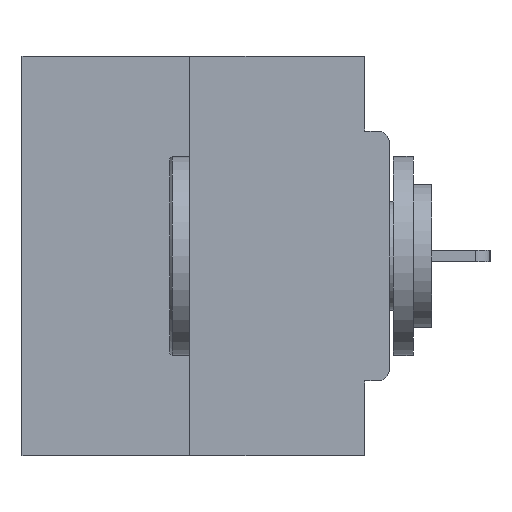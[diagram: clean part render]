
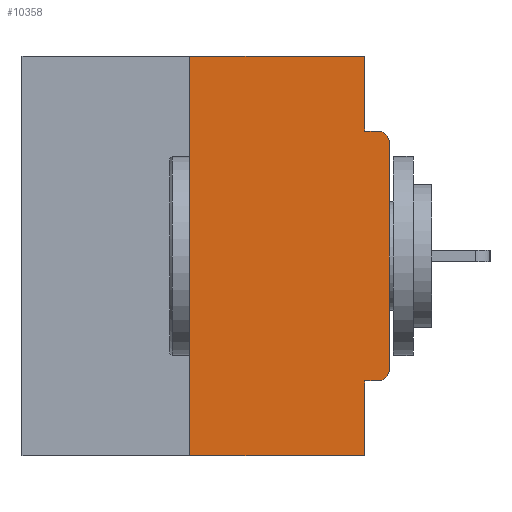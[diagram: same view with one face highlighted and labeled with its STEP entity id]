
A CAD part, left-side view. The second image highlights one B-rep face of the part: STEP entity #10358.
In plain terms, the highlighted planar face has unit normal (-1, 0, 0).
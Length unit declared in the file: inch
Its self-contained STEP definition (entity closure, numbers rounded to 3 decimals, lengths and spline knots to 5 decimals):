
#1266 = DIRECTION ( 'NONE',  ( -1., 0., 0. ) ) ;
#2872 = CARTESIAN_POINT ( 'NONE',  ( 0., 0.46, -0.5 ) ) ;
#3103 = VERTEX_POINT ( 'NONE', #32053 ) ;
#3168 = CARTESIAN_POINT ( 'NONE',  ( 0., 0., -0.4065 ) ) ;
#3614 = ORIENTED_EDGE ( 'NONE', *, *, #15374, .F. ) ;
#3840 = CARTESIAN_POINT ( 'NONE',  ( 0., 0.46, 0. ) ) ;
#3974 = LINE ( 'NONE', #3168, #19905 ) ;
#4709 = AXIS2_PLACEMENT_3D ( 'NONE', #33592, #14643, #36717 ) ;
#5144 = ORIENTED_EDGE ( 'NONE', *, *, #16785, .T. ) ;
#6228 = EDGE_CURVE ( 'NONE', #33086, #18322, #9786, .T. ) ;
#6439 = DIRECTION ( 'NONE',  ( 0., 1., 0. ) ) ;
#6681 = ORIENTED_EDGE ( 'NONE', *, *, #34825, .F. ) ;
#7088 = CARTESIAN_POINT ( 'NONE',  ( 0., 0.031, -0.4065 ) ) ;
#7134 = EDGE_CURVE ( 'NONE', #12726, #3103, #34498, .T. ) ;
#7839 = DIRECTION ( 'NONE',  ( 0., 0., -1. ) ) ;
#7960 = DIRECTION ( 'NONE',  ( 1., 0., 0. ) ) ;
#8054 = VECTOR ( 'NONE', #36622, 39.37008 ) ;
#8109 = PLANE ( 'NONE',  #19011 ) ;
#8117 = CARTESIAN_POINT ( 'NONE',  ( 0., 0.25, -0.5 ) ) ;
#8570 = VECTOR ( 'NONE', #26077, 39.37008 ) ;
#8656 = VERTEX_POINT ( 'NONE', #17662 ) ;
#8841 = CARTESIAN_POINT ( 'NONE',  ( 0., 0.46, 0. ) ) ;
#9786 = LINE ( 'NONE', #16231, #26636 ) ;
#10123 = CARTESIAN_POINT ( 'NONE',  ( 0., 0.031, 0. ) ) ;
#10236 = LINE ( 'NONE', #14665, #34460 ) ;
#10358 = ADVANCED_FACE ( 'NONE', ( #35664 ), #8109, .F. ) ;
#10622 = VERTEX_POINT ( 'NONE', #30970 ) ;
#11756 = VERTEX_POINT ( 'NONE', #8117 ) ;
#12726 = VERTEX_POINT ( 'NONE', #28962 ) ;
#13020 = EDGE_CURVE ( 'NONE', #3103, #8656, #40274, .T. ) ;
#14555 = CARTESIAN_POINT ( 'NONE',  ( 0., 0., -0.0935 ) ) ;
#14591 = ORIENTED_EDGE ( 'NONE', *, *, #39870, .F. ) ;
#14643 = DIRECTION ( 'NONE',  ( -1., 0., 0. ) ) ;
#14665 = CARTESIAN_POINT ( 'NONE',  ( 0., 0.25, 0. ) ) ;
#14798 = CARTESIAN_POINT ( 'NONE',  ( 0., 0.031, 0. ) ) ;
#15153 = EDGE_CURVE ( 'NONE', #22543, #38766, #24403, .T. ) ;
#15210 = CIRCLE ( 'NONE', #15786, 0.015 ) ;
#15374 = EDGE_CURVE ( 'NONE', #10622, #8656, #32279, .T. ) ;
#15508 = DIRECTION ( 'NONE',  ( 0., 0., -1. ) ) ;
#15786 = AXIS2_PLACEMENT_3D ( 'NONE', #20370, #1266, #23510 ) ;
#16231 = CARTESIAN_POINT ( 'NONE',  ( 0., 0.031, -0.5 ) ) ;
#16785 = EDGE_CURVE ( 'NONE', #11756, #18322, #22345, .T. ) ;
#17662 = CARTESIAN_POINT ( 'NONE',  ( 0., 0.015, -0.0935 ) ) ;
#18322 = VERTEX_POINT ( 'NONE', #23068 ) ;
#19011 = AXIS2_PLACEMENT_3D ( 'NONE', #8841, #7960, #7839 ) ;
#19040 = ORIENTED_EDGE ( 'NONE', *, *, #15153, .F. ) ;
#19469 = CARTESIAN_POINT ( 'NONE',  ( 0., 0., 0. ) ) ;
#19706 = DIRECTION ( 'NONE',  ( 0., 0., 1. ) ) ;
#19905 = VECTOR ( 'NONE', #6439, 39.37008 ) ;
#20370 = CARTESIAN_POINT ( 'NONE',  ( 0., 0.015, -0.3915 ) ) ;
#22345 = LINE ( 'NONE', #2872, #28815 ) ;
#22543 = VERTEX_POINT ( 'NONE', #29124 ) ;
#23068 = CARTESIAN_POINT ( 'NONE',  ( 0., 0.031, -0.5 ) ) ;
#23510 = DIRECTION ( 'NONE',  ( 0., 0., -1. ) ) ;
#24403 = LINE ( 'NONE', #3840, #8570 ) ;
#24852 = EDGE_LOOP ( 'NONE', ( #19040, #36791, #5144, #38727, #14591, #40645, #33386, #35330, #3614, #6681 ) ) ;
#26077 = DIRECTION ( 'NONE',  ( 0., -1., 0. ) ) ;
#26139 = VECTOR ( 'NONE', #19706, 39.37008 ) ;
#26195 = CARTESIAN_POINT ( 'NONE',  ( 0., 0.015, -0.4065 ) ) ;
#26636 = VECTOR ( 'NONE', #15508, 39.37008 ) ;
#28815 = VECTOR ( 'NONE', #40700, 39.37008 ) ;
#28962 = CARTESIAN_POINT ( 'NONE',  ( 0., 0., -0.3915 ) ) ;
#29124 = CARTESIAN_POINT ( 'NONE',  ( 0., 0.25, 0. ) ) ;
#29429 = VECTOR ( 'NONE', #33740, 39.37008 ) ;
#30970 = CARTESIAN_POINT ( 'NONE',  ( 0., 0.031, -0.0935 ) ) ;
#30989 = VERTEX_POINT ( 'NONE', #26195 ) ;
#32053 = CARTESIAN_POINT ( 'NONE',  ( 0., 0., -0.1085 ) ) ;
#32279 = LINE ( 'NONE', #14555, #8054 ) ;
#33086 = VERTEX_POINT ( 'NONE', #7088 ) ;
#33386 = ORIENTED_EDGE ( 'NONE', *, *, #7134, .T. ) ;
#33592 = CARTESIAN_POINT ( 'NONE',  ( 0., 0.015, -0.1085 ) ) ;
#33740 = DIRECTION ( 'NONE',  ( 0., 0., -1. ) ) ;
#34460 = VECTOR ( 'NONE', #36737, 39.37008 ) ;
#34498 = LINE ( 'NONE', #19469, #26139 ) ;
#34825 = EDGE_CURVE ( 'NONE', #38766, #10622, #36761, .T. ) ;
#35330 = ORIENTED_EDGE ( 'NONE', *, *, #13020, .T. ) ;
#35664 = FACE_OUTER_BOUND ( 'NONE', #24852, .T. ) ;
#36413 = EDGE_CURVE ( 'NONE', #30989, #12726, #15210, .T. ) ;
#36540 = EDGE_CURVE ( 'NONE', #11756, #22543, #10236, .T. ) ;
#36622 = DIRECTION ( 'NONE',  ( 0., -1., 0. ) ) ;
#36717 = DIRECTION ( 'NONE',  ( 0., 0., -1. ) ) ;
#36737 = DIRECTION ( 'NONE',  ( 0., 0., 1. ) ) ;
#36761 = LINE ( 'NONE', #14798, #29429 ) ;
#36791 = ORIENTED_EDGE ( 'NONE', *, *, #36540, .F. ) ;
#38727 = ORIENTED_EDGE ( 'NONE', *, *, #6228, .F. ) ;
#38766 = VERTEX_POINT ( 'NONE', #10123 ) ;
#39870 = EDGE_CURVE ( 'NONE', #30989, #33086, #3974, .T. ) ;
#40274 = CIRCLE ( 'NONE', #4709, 0.015 ) ;
#40645 = ORIENTED_EDGE ( 'NONE', *, *, #36413, .T. ) ;
#40700 = DIRECTION ( 'NONE',  ( 0., -1., 0. ) ) ;
